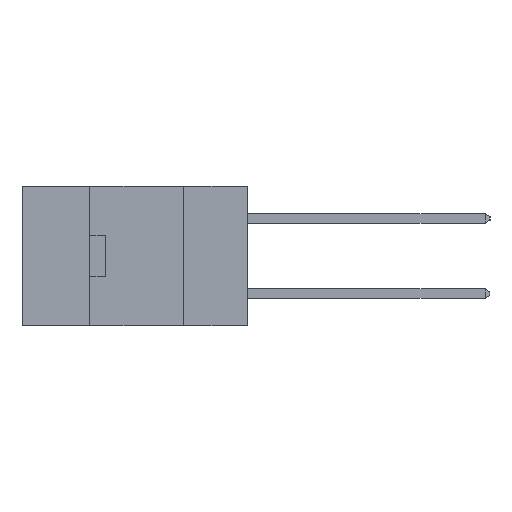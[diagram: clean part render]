
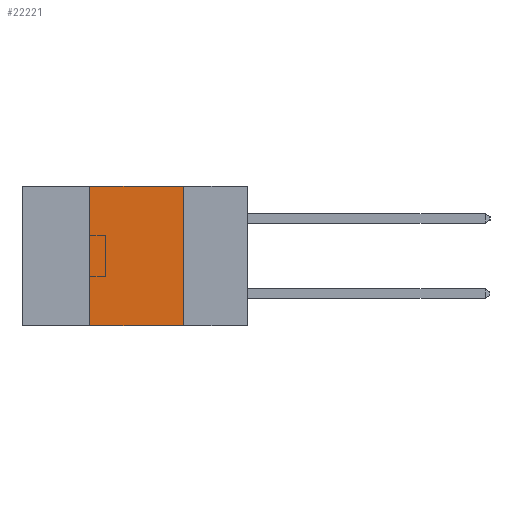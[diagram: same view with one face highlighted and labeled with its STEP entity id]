
A CAD part, left-side view. The second image highlights one B-rep face of the part: STEP entity #22221.
In plain terms, the highlighted planar face has unit normal (-1, 0, 0).
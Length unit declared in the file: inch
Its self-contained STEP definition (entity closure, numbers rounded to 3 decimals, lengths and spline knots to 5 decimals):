
#196 = LINE ( 'NONE', #8890, #27952 ) ;
#1981 = CARTESIAN_POINT ( 'NONE',  ( 0., 0.42, -0.37 ) ) ;
#2130 = VERTEX_POINT ( 'NONE', #1981 ) ;
#3123 = DIRECTION ( 'NONE',  ( 0., 0., -1. ) ) ;
#3834 = DIRECTION ( 'NONE',  ( 0., 0., 1. ) ) ;
#4510 = DIRECTION ( 'NONE',  ( 0., -1., 0. ) ) ;
#5087 = ORIENTED_EDGE ( 'NONE', *, *, #24337, .T. ) ;
#6170 = DIRECTION ( 'NONE',  ( 0., 0., -1. ) ) ;
#6773 = AXIS2_PLACEMENT_3D ( 'NONE', #17126, #19318, #6170 ) ;
#8669 = CARTESIAN_POINT ( 'NONE',  ( 0., 0.6, -0.37 ) ) ;
#8890 = CARTESIAN_POINT ( 'NONE',  ( 0., 0.17, -0.37 ) ) ;
#9198 = EDGE_LOOP ( 'NONE', ( #14639, #21841, #14033, #5087 ) ) ;
#10527 = CARTESIAN_POINT ( 'NONE',  ( 0., 0.42, -0.37 ) ) ;
#12683 = EDGE_CURVE ( 'NONE', #16441, #12921, #196, .T. ) ;
#12921 = VERTEX_POINT ( 'NONE', #16142 ) ;
#14033 = ORIENTED_EDGE ( 'NONE', *, *, #22857, .F. ) ;
#14611 = VERTEX_POINT ( 'NONE', #18643 ) ;
#14639 = ORIENTED_EDGE ( 'NONE', *, *, #12683, .F. ) ;
#14950 = PLANE ( 'NONE',  #6773 ) ;
#15459 = LINE ( 'NONE', #10527, #21210 ) ;
#15606 = EDGE_CURVE ( 'NONE', #14611, #16441, #28118, .T. ) ;
#15857 = FACE_OUTER_BOUND ( 'NONE', #9198, .T. ) ;
#16142 = CARTESIAN_POINT ( 'NONE',  ( 0., 0.17, -0.37 ) ) ;
#16441 = VERTEX_POINT ( 'NONE', #22551 ) ;
#17126 = CARTESIAN_POINT ( 'NONE',  ( 0., 0.6, 0. ) ) ;
#18643 = CARTESIAN_POINT ( 'NONE',  ( 0., 0.42, 0. ) ) ;
#19318 = DIRECTION ( 'NONE',  ( 1., 0., 0. ) ) ;
#19774 = CARTESIAN_POINT ( 'NONE',  ( 0., 0.6, 0. ) ) ;
#21210 = VECTOR ( 'NONE', #3834, 39.37008 ) ;
#21722 = DIRECTION ( 'NONE',  ( 0., -1., 0. ) ) ;
#21841 = ORIENTED_EDGE ( 'NONE', *, *, #15606, .F. ) ;
#22221 = ADVANCED_FACE ( 'NONE', ( #15857 ), #14950, .F. ) ;
#22383 = VECTOR ( 'NONE', #4510, 39.37008 ) ;
#22551 = CARTESIAN_POINT ( 'NONE',  ( 0., 0.17, 0. ) ) ;
#22772 = LINE ( 'NONE', #8669, #24162 ) ;
#22857 = EDGE_CURVE ( 'NONE', #2130, #14611, #15459, .T. ) ;
#24162 = VECTOR ( 'NONE', #21722, 39.37008 ) ;
#24337 = EDGE_CURVE ( 'NONE', #2130, #12921, #22772, .T. ) ;
#27952 = VECTOR ( 'NONE', #3123, 39.37008 ) ;
#28118 = LINE ( 'NONE', #19774, #22383 ) ;
